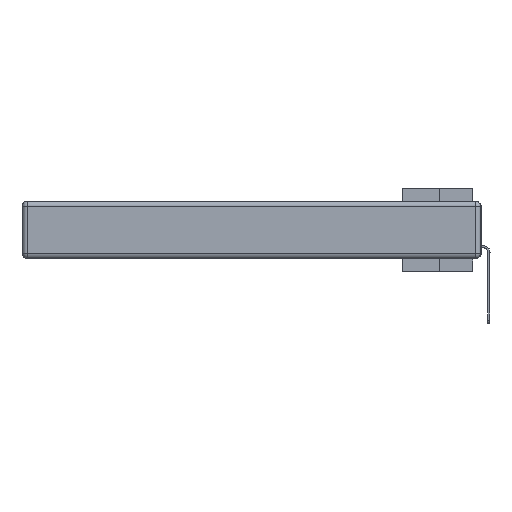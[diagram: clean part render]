
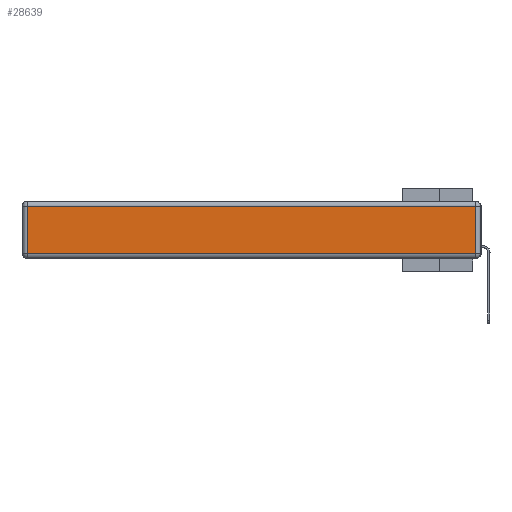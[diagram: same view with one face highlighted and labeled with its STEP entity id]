
A CAD part, left-side view. The second image highlights one B-rep face of the part: STEP entity #28639.
In plain terms, the highlighted planar face has unit normal (-1, 0, 0).
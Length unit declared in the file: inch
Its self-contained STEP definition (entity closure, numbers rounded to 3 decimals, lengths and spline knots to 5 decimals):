
#53 = CARTESIAN_POINT ( 'NONE',  ( 0., 2.75, -0.03 ) ) ;
#867 = CARTESIAN_POINT ( 'NONE',  ( 0., 0., -0.313 ) ) ;
#1136 = VECTOR ( 'NONE', #19385, 39.37008 ) ;
#1508 = CARTESIAN_POINT ( 'NONE',  ( 0., 0.03, -0.313 ) ) ;
#4040 = DIRECTION ( 'NONE',  ( 0., 0., 1. ) ) ;
#4185 = CARTESIAN_POINT ( 'NONE',  ( 0., 0.03, -0.03 ) ) ;
#4831 = ORIENTED_EDGE ( 'NONE', *, *, #12635, .T. ) ;
#5530 = CARTESIAN_POINT ( 'NONE',  ( 0., 2.72, -0.03 ) ) ;
#8923 = ORIENTED_EDGE ( 'NONE', *, *, #12303, .T. ) ;
#9426 = LINE ( 'NONE', #53, #1136 ) ;
#9764 = VERTEX_POINT ( 'NONE', #5530 ) ;
#10076 = VERTEX_POINT ( 'NONE', #26922 ) ;
#10390 = VERTEX_POINT ( 'NONE', #4185 ) ;
#11127 = DIRECTION ( 'NONE',  ( 0., 0., 1. ) ) ;
#11585 = EDGE_CURVE ( 'NONE', #10390, #9764, #9426, .T. ) ;
#12303 = EDGE_CURVE ( 'NONE', #10076, #27362, #22131, .T. ) ;
#12635 = EDGE_CURVE ( 'NONE', #9764, #10076, #31023, .T. ) ;
#16577 = PLANE ( 'NONE',  #28800 ) ;
#16979 = ORIENTED_EDGE ( 'NONE', *, *, #20409, .T. ) ;
#18223 = EDGE_LOOP ( 'NONE', ( #8923, #16979, #28789, #4831 ) ) ;
#19385 = DIRECTION ( 'NONE',  ( 0., 1., 0. ) ) ;
#20365 = DIRECTION ( 'NONE',  ( 0., -1., 0. ) ) ;
#20409 = EDGE_CURVE ( 'NONE', #27362, #10390, #25931, .T. ) ;
#22131 = LINE ( 'NONE', #867, #30770 ) ;
#22407 = VECTOR ( 'NONE', #4040, 39.37008 ) ;
#25691 = CARTESIAN_POINT ( 'NONE',  ( 0., 0., -0.343 ) ) ;
#25931 = LINE ( 'NONE', #28356, #22407 ) ;
#26922 = CARTESIAN_POINT ( 'NONE',  ( 0., 2.72, -0.313 ) ) ;
#27362 = VERTEX_POINT ( 'NONE', #1508 ) ;
#28356 = CARTESIAN_POINT ( 'NONE',  ( 0., 0.03, -0.343 ) ) ;
#28423 = DIRECTION ( 'NONE',  ( -1., 0., 0. ) ) ;
#28493 = CARTESIAN_POINT ( 'NONE',  ( 0., 2.72, -0.343 ) ) ;
#28639 = ADVANCED_FACE ( 'NONE', ( #30953 ), #16577, .T. ) ;
#28789 = ORIENTED_EDGE ( 'NONE', *, *, #11585, .T. ) ;
#28800 = AXIS2_PLACEMENT_3D ( 'NONE', #25691, #28423, #11127 ) ;
#29249 = VECTOR ( 'NONE', #31178, 39.37008 ) ;
#30770 = VECTOR ( 'NONE', #20365, 39.37008 ) ;
#30953 = FACE_OUTER_BOUND ( 'NONE', #18223, .T. ) ;
#31023 = LINE ( 'NONE', #28493, #29249 ) ;
#31178 = DIRECTION ( 'NONE',  ( 0., 0., -1. ) ) ;
